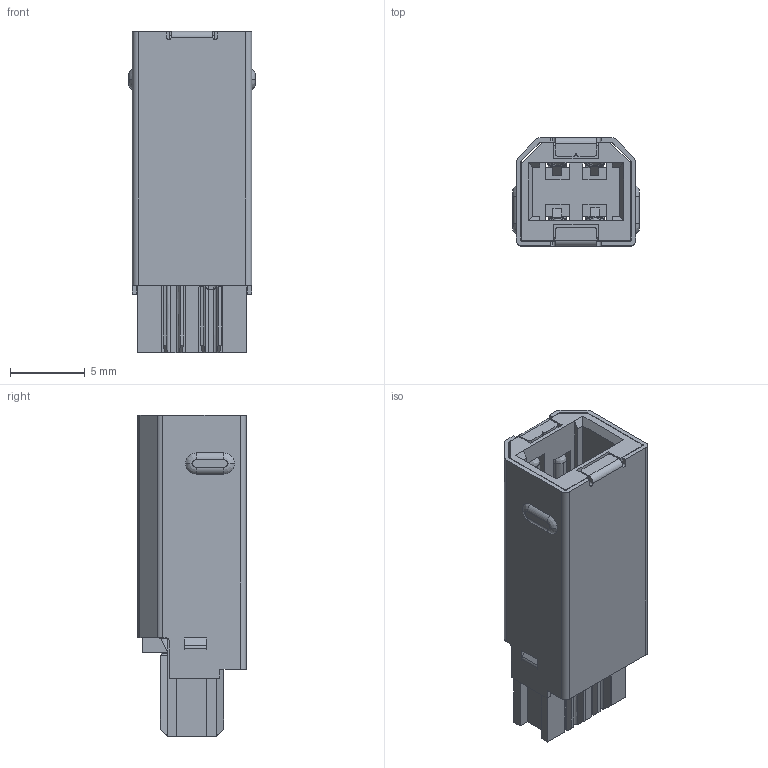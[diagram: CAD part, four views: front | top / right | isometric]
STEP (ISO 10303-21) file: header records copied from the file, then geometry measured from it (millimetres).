
FILE_DESCRIPTION (( 'STEP AP214' ), '1' );
FILE_NAME ('691F204-190-120.STEP', '2021-01-19T14:53:44', ( '' ), ( '' ), 'SwSTEP 2.0', 'SolidWorks 2020', '' );
FILE_SCHEMA (( 'AUTOMOTIVE_DESIGN' ));
Length unit declared in the file: millimetre
Products named in the file (5): Contact2 691F204-X90-12X; 691F204-190-120; Insulator 691F204-X90-12X_White; Contact1 691F204-X90-12X; Shell 691F204-X90-12X
Assembly tree (6 placements, depth 2):
  691F204-190-120
    Insulator 691F204-X90-12X_White
    Contact2 691F204-X90-12X  x2
    Shell 691F204-X90-12X
    Contact1 691F204-X90-12X  x2
Bounding box: 8.5 x 7.26 x 21.51 mm (x, y, z)
Volume: 709.4 mm3; surface area: 2337.4 mm2
Topology: 6 solids, 6 shells, 865 faces, 2164 edges, 1282 vertices
Faces by surface type: plane 425, bspline 324, cylinder 116
Entity records: 24025 total; most frequent: CARTESIAN_POINT 12091, ORIENTED_EDGE 2842, DIRECTION 1800, EDGE_CURVE 1421, VERTEX_POINT 861, LINE 790, VECTOR 790, EDGE_LOOP 564
